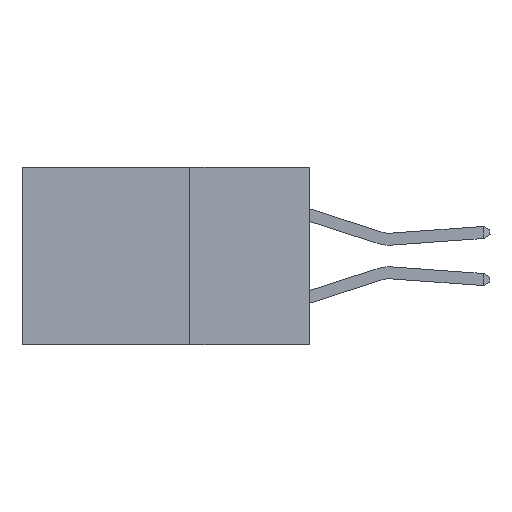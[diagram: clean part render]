
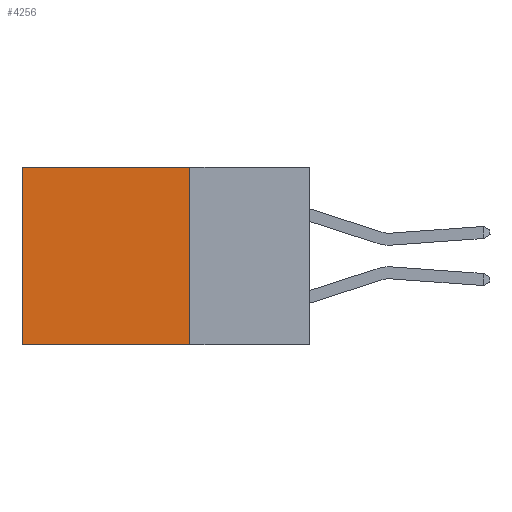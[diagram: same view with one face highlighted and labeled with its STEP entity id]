
A CAD part, left-side view. The second image highlights one B-rep face of the part: STEP entity #4256.
In plain terms, the highlighted planar face has unit normal (-1, 0, 0).
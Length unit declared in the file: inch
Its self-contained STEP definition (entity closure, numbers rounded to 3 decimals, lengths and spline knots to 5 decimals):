
#252 = DIRECTION ( 'NONE',  ( 1., 0., 0. ) ) ;
#458 = EDGE_CURVE ( 'NONE', #9783, #850, #2691, .T. ) ;
#522 = ORIENTED_EDGE ( 'NONE', *, *, #3394, .F. ) ;
#548 = CARTESIAN_POINT ( 'NONE',  ( 0.2615, 0.25, -0.37 ) ) ;
#850 = VERTEX_POINT ( 'NONE', #886 ) ;
#886 = CARTESIAN_POINT ( 'NONE',  ( 0.2615, 0.6, 0. ) ) ;
#1155 = EDGE_CURVE ( 'NONE', #6115, #9583, #4013, .T. ) ;
#1691 = VECTOR ( 'NONE', #1989, 39.37008 ) ;
#1732 = VECTOR ( 'NONE', #7626, 39.37008 ) ;
#1989 = DIRECTION ( 'NONE',  ( 0., 0., -1. ) ) ;
#2396 = CARTESIAN_POINT ( 'NONE',  ( 0.2615, 0.25, 0. ) ) ;
#2420 = VECTOR ( 'NONE', #3623, 39.37008 ) ;
#2570 = EDGE_LOOP ( 'NONE', ( #4713, #7044, #522, #6598 ) ) ;
#2691 = LINE ( 'NONE', #5197, #2420 ) ;
#2746 = PLANE ( 'NONE',  #6887 ) ;
#3394 = EDGE_CURVE ( 'NONE', #9783, #6115, #8297, .T. ) ;
#3623 = DIRECTION ( 'NONE',  ( 0., 1., 0. ) ) ;
#3883 = CARTESIAN_POINT ( 'NONE',  ( 0.2615, 0.25, -0.37 ) ) ;
#4013 = LINE ( 'NONE', #8928, #1732 ) ;
#4256 = ADVANCED_FACE ( 'NONE', ( #8155 ), #2746, .F. ) ;
#4713 = ORIENTED_EDGE ( 'NONE', *, *, #9372, .T. ) ;
#5197 = CARTESIAN_POINT ( 'NONE',  ( 0.2615, 0.25, 0. ) ) ;
#5726 = LINE ( 'NONE', #7345, #1691 ) ;
#5879 = DIRECTION ( 'NONE',  ( 0., 0., -1. ) ) ;
#6115 = VERTEX_POINT ( 'NONE', #548 ) ;
#6231 = VECTOR ( 'NONE', #8891, 39.37008 ) ;
#6598 = ORIENTED_EDGE ( 'NONE', *, *, #458, .T. ) ;
#6887 = AXIS2_PLACEMENT_3D ( 'NONE', #8641, #252, #5879 ) ;
#7044 = ORIENTED_EDGE ( 'NONE', *, *, #1155, .F. ) ;
#7345 = CARTESIAN_POINT ( 'NONE',  ( 0.2615, 0.6, -0.37 ) ) ;
#7626 = DIRECTION ( 'NONE',  ( 0., 1., 0. ) ) ;
#8155 = FACE_OUTER_BOUND ( 'NONE', #2570, .T. ) ;
#8297 = LINE ( 'NONE', #3883, #6231 ) ;
#8641 = CARTESIAN_POINT ( 'NONE',  ( 0.2615, 0.25, -0.37 ) ) ;
#8891 = DIRECTION ( 'NONE',  ( 0., 0., -1. ) ) ;
#8928 = CARTESIAN_POINT ( 'NONE',  ( 0.2615, 0.25, -0.37 ) ) ;
#9372 = EDGE_CURVE ( 'NONE', #850, #9583, #5726, .T. ) ;
#9534 = CARTESIAN_POINT ( 'NONE',  ( 0.2615, 0.6, -0.37 ) ) ;
#9583 = VERTEX_POINT ( 'NONE', #9534 ) ;
#9783 = VERTEX_POINT ( 'NONE', #2396 ) ;
